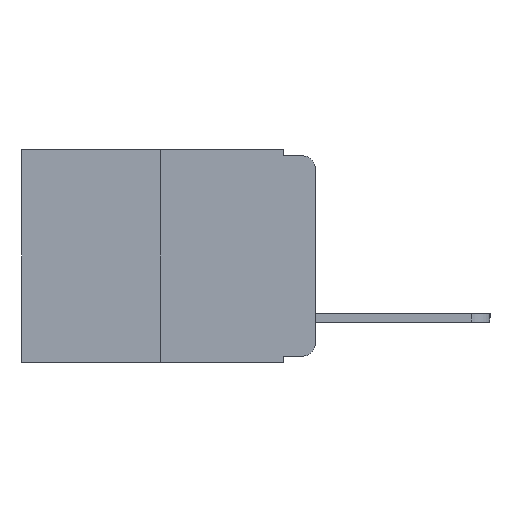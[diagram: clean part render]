
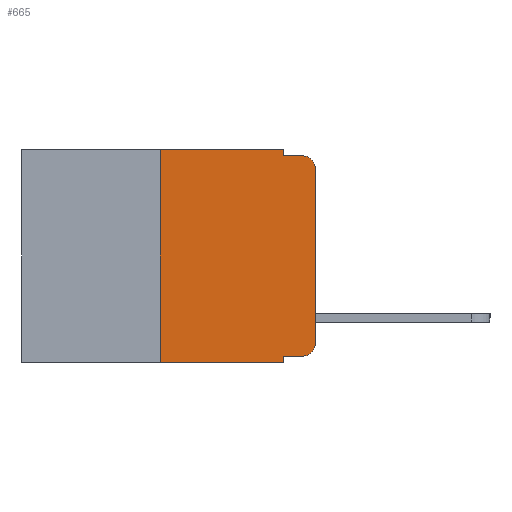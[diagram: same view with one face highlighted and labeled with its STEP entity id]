
A CAD part, left-side view. The second image highlights one B-rep face of the part: STEP entity #665.
In plain terms, the highlighted planar face has unit normal (-1, 0, 0).
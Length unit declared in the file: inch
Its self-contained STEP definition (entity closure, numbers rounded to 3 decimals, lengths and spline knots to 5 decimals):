
#207 = CARTESIAN_POINT ( 'NONE',  ( 0., 0.051, 0. ) ) ;
#665 = ADVANCED_FACE ( 'NONE', ( #9926 ), #4098, .F. ) ;
#796 = DIRECTION ( 'NONE',  ( 1., 0., 0. ) ) ;
#808 = CARTESIAN_POINT ( 'NONE',  ( 0., 0.25, 0. ) ) ;
#1208 = VERTEX_POINT ( 'NONE', #5322 ) ;
#1326 = DIRECTION ( 'NONE',  ( 0., 0., -1. ) ) ;
#1437 = VECTOR ( 'NONE', #17001, 39.37008 ) ;
#2040 = LINE ( 'NONE', #7869, #1437 ) ;
#2157 = CARTESIAN_POINT ( 'NONE',  ( 0., 0.02, -0.03 ) ) ;
#2200 = VECTOR ( 'NONE', #4287, 39.37008 ) ;
#3233 = EDGE_CURVE ( 'NONE', #3286, #5419, #2040, .T. ) ;
#3286 = VERTEX_POINT ( 'NONE', #808 ) ;
#3945 = CARTESIAN_POINT ( 'NONE',  ( 0., 0.02, -0.313 ) ) ;
#4045 = DIRECTION ( 'NONE',  ( 0., 0., -1. ) ) ;
#4098 = PLANE ( 'NONE',  #16092 ) ;
#4261 = EDGE_CURVE ( 'NONE', #7294, #9134, #16513, .T. ) ;
#4287 = DIRECTION ( 'NONE',  ( 0., 0., 1. ) ) ;
#5322 = CARTESIAN_POINT ( 'NONE',  ( 0., 0.051, -0.333 ) ) ;
#5419 = VERTEX_POINT ( 'NONE', #8165 ) ;
#5473 = EDGE_CURVE ( 'NONE', #1208, #7294, #14084, .T. ) ;
#5730 = DIRECTION ( 'NONE',  ( 0., 0., -1. ) ) ;
#5757 = EDGE_CURVE ( 'NONE', #10268, #7147, #8362, .T. ) ;
#6155 = VECTOR ( 'NONE', #8377, 39.37008 ) ;
#6208 = CARTESIAN_POINT ( 'NONE',  ( 0., 0.25, -0.343 ) ) ;
#6459 = VERTEX_POINT ( 'NONE', #10198 ) ;
#6611 = CARTESIAN_POINT ( 'NONE',  ( 0., 0.051, -0.333 ) ) ;
#6636 = EDGE_CURVE ( 'NONE', #1208, #7147, #11777, .T. ) ;
#7135 = LINE ( 'NONE', #8501, #14898 ) ;
#7147 = VERTEX_POINT ( 'NONE', #16926 ) ;
#7294 = VERTEX_POINT ( 'NONE', #12764 ) ;
#7686 = DIRECTION ( 'NONE',  ( 0., -1., 0. ) ) ;
#7716 = CARTESIAN_POINT ( 'NONE',  ( 0., 0., -0.03 ) ) ;
#7815 = VECTOR ( 'NONE', #7686, 39.37008 ) ;
#7823 = EDGE_CURVE ( 'NONE', #10268, #3286, #11695, .T. ) ;
#7869 = CARTESIAN_POINT ( 'NONE',  ( 0., 0.473, 0. ) ) ;
#8000 = CARTESIAN_POINT ( 'NONE',  ( 0., 0.051, -0.01 ) ) ;
#8165 = CARTESIAN_POINT ( 'NONE',  ( 0., 0.051, 0. ) ) ;
#8183 = VERTEX_POINT ( 'NONE', #12016 ) ;
#8362 = LINE ( 'NONE', #12202, #7815 ) ;
#8377 = DIRECTION ( 'NONE',  ( 0., -1., 0. ) ) ;
#8501 = CARTESIAN_POINT ( 'NONE',  ( 0., 0.051, 0. ) ) ;
#8933 = EDGE_CURVE ( 'NONE', #5419, #6459, #7135, .T. ) ;
#9134 = VERTEX_POINT ( 'NONE', #13469 ) ;
#9301 = EDGE_LOOP ( 'NONE', ( #13556, #12014, #19254, #18286, #18142, #18103, #18049, #16252, #14826, #14137 ) ) ;
#9320 = AXIS2_PLACEMENT_3D ( 'NONE', #3945, #15200, #5730 ) ;
#9926 = FACE_OUTER_BOUND ( 'NONE', #9301, .T. ) ;
#9976 = DIRECTION ( 'NONE',  ( 0., 0., -1. ) ) ;
#10198 = CARTESIAN_POINT ( 'NONE',  ( 0., 0.051, -0.01 ) ) ;
#10268 = VERTEX_POINT ( 'NONE', #6208 ) ;
#10361 = CARTESIAN_POINT ( 'NONE',  ( 0., 0., 0. ) ) ;
#10660 = DIRECTION ( 'NONE',  ( 0., 0., -1. ) ) ;
#10721 = VECTOR ( 'NONE', #12615, 39.37008 ) ;
#10810 = VECTOR ( 'NONE', #10660, 39.37008 ) ;
#11695 = LINE ( 'NONE', #13903, #2200 ) ;
#11742 = LINE ( 'NONE', #10361, #19212 ) ;
#11777 = LINE ( 'NONE', #207, #10810 ) ;
#11875 = DIRECTION ( 'NONE',  ( 0., 0., 1. ) ) ;
#11953 = EDGE_CURVE ( 'NONE', #6459, #8183, #15267, .T. ) ;
#12014 = ORIENTED_EDGE ( 'NONE', *, *, #12991, .T. ) ;
#12016 = CARTESIAN_POINT ( 'NONE',  ( 0., 0.02, -0.01 ) ) ;
#12202 = CARTESIAN_POINT ( 'NONE',  ( 0., 0.473, -0.343 ) ) ;
#12615 = DIRECTION ( 'NONE',  ( 0., -1., 0. ) ) ;
#12764 = CARTESIAN_POINT ( 'NONE',  ( 0., 0.02, -0.333 ) ) ;
#12991 = EDGE_CURVE ( 'NONE', #19404, #8183, #13738, .T. ) ;
#13469 = CARTESIAN_POINT ( 'NONE',  ( 0., 0., -0.313 ) ) ;
#13556 = ORIENTED_EDGE ( 'NONE', *, *, #15027, .T. ) ;
#13738 = CIRCLE ( 'NONE', #18762, 0.02 ) ;
#13746 = DIRECTION ( 'NONE',  ( -1., 0., 0. ) ) ;
#13903 = CARTESIAN_POINT ( 'NONE',  ( 0., 0.25, 0. ) ) ;
#14084 = LINE ( 'NONE', #6611, #6155 ) ;
#14137 = ORIENTED_EDGE ( 'NONE', *, *, #4261, .T. ) ;
#14826 = ORIENTED_EDGE ( 'NONE', *, *, #5473, .T. ) ;
#14898 = VECTOR ( 'NONE', #1326, 39.37008 ) ;
#15027 = EDGE_CURVE ( 'NONE', #9134, #19404, #11742, .T. ) ;
#15200 = DIRECTION ( 'NONE',  ( -1., 0., 0. ) ) ;
#15267 = LINE ( 'NONE', #8000, #10721 ) ;
#16092 = AXIS2_PLACEMENT_3D ( 'NONE', #20275, #796, #9976 ) ;
#16252 = ORIENTED_EDGE ( 'NONE', *, *, #6636, .F. ) ;
#16513 = CIRCLE ( 'NONE', #9320, 0.02 ) ;
#16926 = CARTESIAN_POINT ( 'NONE',  ( 0., 0.051, -0.343 ) ) ;
#17001 = DIRECTION ( 'NONE',  ( 0., -1., 0. ) ) ;
#18049 = ORIENTED_EDGE ( 'NONE', *, *, #5757, .T. ) ;
#18103 = ORIENTED_EDGE ( 'NONE', *, *, #7823, .F. ) ;
#18142 = ORIENTED_EDGE ( 'NONE', *, *, #3233, .F. ) ;
#18286 = ORIENTED_EDGE ( 'NONE', *, *, #8933, .F. ) ;
#18762 = AXIS2_PLACEMENT_3D ( 'NONE', #2157, #13746, #4045 ) ;
#19212 = VECTOR ( 'NONE', #11875, 39.37008 ) ;
#19254 = ORIENTED_EDGE ( 'NONE', *, *, #11953, .F. ) ;
#19404 = VERTEX_POINT ( 'NONE', #7716 ) ;
#20275 = CARTESIAN_POINT ( 'NONE',  ( 0., 0.473, 0. ) ) ;
